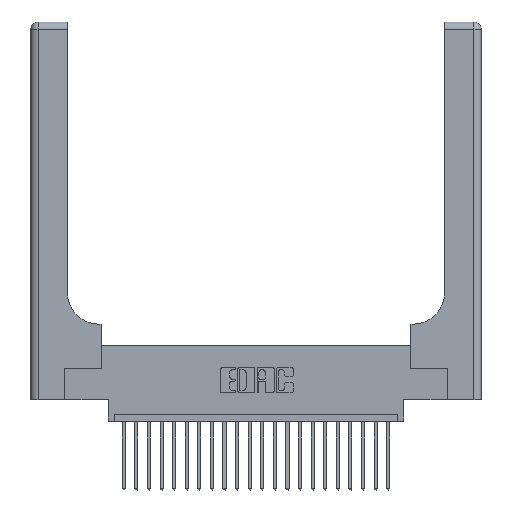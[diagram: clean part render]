
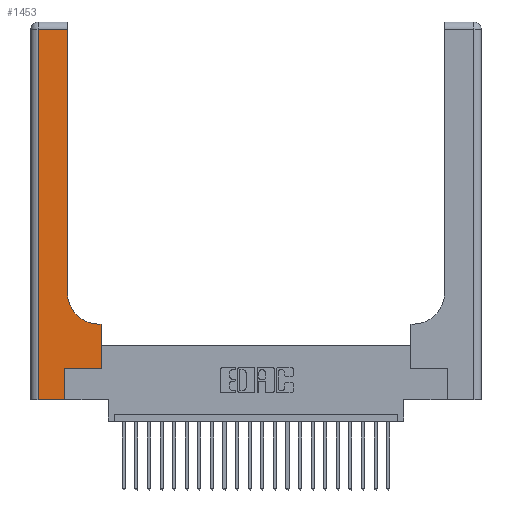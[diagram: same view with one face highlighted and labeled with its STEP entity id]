
A CAD part, top view. The second image highlights one B-rep face of the part: STEP entity #1453.
In plain terms, the highlighted planar face has unit normal (0, 0, 1).
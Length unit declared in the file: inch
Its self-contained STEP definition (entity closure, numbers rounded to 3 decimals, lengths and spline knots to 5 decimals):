
#536 = CARTESIAN_POINT ( 'NONE',  ( 0.06, 0., 0.37 ) ) ;
#1161 = VERTEX_POINT ( 'NONE', #16750 ) ;
#1453 = ADVANCED_FACE ( 'NONE', ( #1913 ), #4677, .F. ) ;
#1913 = FACE_OUTER_BOUND ( 'NONE', #16870, .T. ) ;
#2038 = ORIENTED_EDGE ( 'NONE', *, *, #13857, .T. ) ;
#2177 = ORIENTED_EDGE ( 'NONE', *, *, #9595, .T. ) ;
#2246 = ORIENTED_EDGE ( 'NONE', *, *, #9370, .T. ) ;
#2295 = LINE ( 'NONE', #21755, #18048 ) ;
#2400 = LINE ( 'NONE', #5568, #22005 ) ;
#2636 = DIRECTION ( 'NONE',  ( 0., 1., 0. ) ) ;
#2638 = DIRECTION ( 'NONE',  ( 1., 0., 0. ) ) ;
#2832 = CARTESIAN_POINT ( 'NONE',  ( 0.2915, 0.85, 0.37 ) ) ;
#2880 = DIRECTION ( 'NONE',  ( 0., 0., -1. ) ) ;
#3017 = ORIENTED_EDGE ( 'NONE', *, *, #17670, .T. ) ;
#3950 = EDGE_CURVE ( 'NONE', #13981, #7831, #2400, .T. ) ;
#4139 = VERTEX_POINT ( 'NONE', #2832 ) ;
#4677 = PLANE ( 'NONE',  #10899 ) ;
#5175 = VECTOR ( 'NONE', #2636, 39.37008 ) ;
#5483 = ORIENTED_EDGE ( 'NONE', *, *, #6492, .T. ) ;
#5568 = CARTESIAN_POINT ( 'NONE',  ( 0.5585, 0.25, 0.37 ) ) ;
#5707 = CARTESIAN_POINT ( 'NONE',  ( 0.06, 2.94, 0.37 ) ) ;
#5912 = CARTESIAN_POINT ( 'NONE',  ( 0.5415, 0.85, 0.37 ) ) ;
#6097 = DIRECTION ( 'NONE',  ( -1., 0., 0. ) ) ;
#6342 = CARTESIAN_POINT ( 'NONE',  ( 0., 3., 0.37 ) ) ;
#6460 = CARTESIAN_POINT ( 'NONE',  ( 0., 0., 0.37 ) ) ;
#6492 = EDGE_CURVE ( 'NONE', #15699, #13981, #2295, .T. ) ;
#6510 = VERTEX_POINT ( 'NONE', #6734 ) ;
#6734 = CARTESIAN_POINT ( 'NONE',  ( 0.5415, 0.6, 0.37 ) ) ;
#7537 = LINE ( 'NONE', #23217, #9948 ) ;
#7557 = LINE ( 'NONE', #12214, #5175 ) ;
#7831 = VERTEX_POINT ( 'NONE', #15417 ) ;
#7994 = DIRECTION ( 'NONE',  ( 0., -1., 0. ) ) ;
#8982 = VECTOR ( 'NONE', #2638, 39.37008 ) ;
#9178 = CARTESIAN_POINT ( 'NONE',  ( 0.5585, 0.25, 0.37 ) ) ;
#9370 = EDGE_CURVE ( 'NONE', #4139, #1161, #7557, .T. ) ;
#9515 = CIRCLE ( 'NONE', #22844, 0.25 ) ;
#9595 = EDGE_CURVE ( 'NONE', #1161, #14640, #7537, .T. ) ;
#9948 = VECTOR ( 'NONE', #21616, 39.37008 ) ;
#10899 = AXIS2_PLACEMENT_3D ( 'NONE', #6342, #2880, #17659 ) ;
#11967 = CARTESIAN_POINT ( 'NONE',  ( 0.269, 0., 0.37 ) ) ;
#12178 = CARTESIAN_POINT ( 'NONE',  ( 0.06, 3., 0.37 ) ) ;
#12214 = CARTESIAN_POINT ( 'NONE',  ( 0.2915, 3., 0.37 ) ) ;
#13163 = LINE ( 'NONE', #17409, #20565 ) ;
#13532 = ORIENTED_EDGE ( 'NONE', *, *, #20409, .T. ) ;
#13857 = EDGE_CURVE ( 'NONE', #19626, #21535, #20896, .T. ) ;
#13981 = VERTEX_POINT ( 'NONE', #9178 ) ;
#14640 = VERTEX_POINT ( 'NONE', #5707 ) ;
#15417 = CARTESIAN_POINT ( 'NONE',  ( 0.5585, 0.6, 0.37 ) ) ;
#15507 = CARTESIAN_POINT ( 'NONE',  ( 0.269, 0., 0.37 ) ) ;
#15629 = VECTOR ( 'NONE', #7994, 39.37008 ) ;
#15699 = VERTEX_POINT ( 'NONE', #21093 ) ;
#16113 = ORIENTED_EDGE ( 'NONE', *, *, #20868, .T. ) ;
#16750 = CARTESIAN_POINT ( 'NONE',  ( 0.2915, 2.94, 0.37 ) ) ;
#16870 = EDGE_LOOP ( 'NONE', ( #2246, #2177, #3017, #2038, #13532, #5483, #17372, #17714, #16113 ) ) ;
#17137 = DIRECTION ( 'NONE',  ( 0., 1., 0. ) ) ;
#17372 = ORIENTED_EDGE ( 'NONE', *, *, #3950, .T. ) ;
#17409 = CARTESIAN_POINT ( 'NONE',  ( 0.2915, 0.6, 0.37 ) ) ;
#17479 = DIRECTION ( 'NONE',  ( 0., 1., 0. ) ) ;
#17659 = DIRECTION ( 'NONE',  ( -1., 0., 0. ) ) ;
#17670 = EDGE_CURVE ( 'NONE', #14640, #19626, #20651, .T. ) ;
#17714 = ORIENTED_EDGE ( 'NONE', *, *, #19466, .T. ) ;
#17877 = DIRECTION ( 'NONE',  ( 1., 0., 0. ) ) ;
#18048 = VECTOR ( 'NONE', #17877, 39.37008 ) ;
#18722 = LINE ( 'NONE', #15507, #19030 ) ;
#19030 = VECTOR ( 'NONE', #17479, 39.37008 ) ;
#19458 = DIRECTION ( 'NONE',  ( 1., 0., 0. ) ) ;
#19466 = EDGE_CURVE ( 'NONE', #7831, #6510, #13163, .T. ) ;
#19626 = VERTEX_POINT ( 'NONE', #536 ) ;
#20409 = EDGE_CURVE ( 'NONE', #21535, #15699, #18722, .T. ) ;
#20565 = VECTOR ( 'NONE', #6097, 39.37008 ) ;
#20651 = LINE ( 'NONE', #12178, #15629 ) ;
#20868 = EDGE_CURVE ( 'NONE', #6510, #4139, #9515, .T. ) ;
#20896 = LINE ( 'NONE', #6460, #8982 ) ;
#21093 = CARTESIAN_POINT ( 'NONE',  ( 0.269, 0.25, 0.37 ) ) ;
#21353 = DIRECTION ( 'NONE',  ( 0., 0., -1. ) ) ;
#21535 = VERTEX_POINT ( 'NONE', #11967 ) ;
#21616 = DIRECTION ( 'NONE',  ( -1., 0., 0. ) ) ;
#21755 = CARTESIAN_POINT ( 'NONE',  ( 0.269, 0.25, 0.37 ) ) ;
#22005 = VECTOR ( 'NONE', #17137, 39.37008 ) ;
#22844 = AXIS2_PLACEMENT_3D ( 'NONE', #5912, #21353, #19458 ) ;
#23217 = CARTESIAN_POINT ( 'NONE',  ( 0., 2.94, 0.37 ) ) ;
